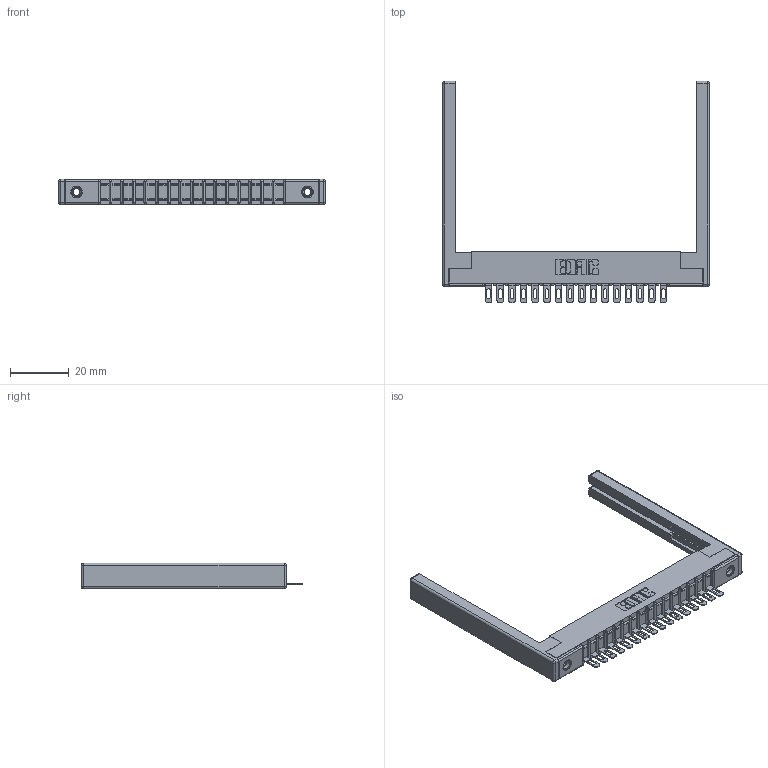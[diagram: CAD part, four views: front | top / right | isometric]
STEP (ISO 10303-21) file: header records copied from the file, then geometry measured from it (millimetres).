
FILE_DESCRIPTION (( 'STEP AP203' ), '1' );
FILE_NAME ('307-016-501-168.STEP', '2019-09-04T21:16:16', ( '' ), ( '' ), 'SwSTEP 2.0', 'SolidWorks 2016', '' );
FILE_SCHEMA (( 'CONFIG_CONTROL_DESIGN' ));
Length unit declared in the file: inch
Products named in the file (5): 345-250-001_345-250-001-102; 307-016-501-168; 307 Part_.156 Dia Mounting Holes; 307-220-068; 307-290-002_501
Assembly tree (21 placements, depth 2):
  307-016-501-168
    307 Part_.156 Dia Mounting Holes
    307-290-002_501  x16
    307-220-068  x2
    345-250-001_345-250-001-102  x2
Bounding box: 90.83 x 75.39 x 8.71 mm (x, y, z)
Volume: 10566 mm3; surface area: 14720.8 mm2
Topology: 21 solids, 21 shells, 1505 faces, 4521 edges, 2946 vertices
Faces by surface type: plane 862, cylinder 585, sphere 42, cone 12, torus 4
Entity records: 20475 total; most frequent: CARTESIAN_POINT 3413, ORIENTED_EDGE 3392, DIRECTION 3350, EDGE_CURVE 1696, LINE 1280, VECTOR 1280, VERTEX_POINT 1098, AXIS2_PLACEMENT_3D 1035
